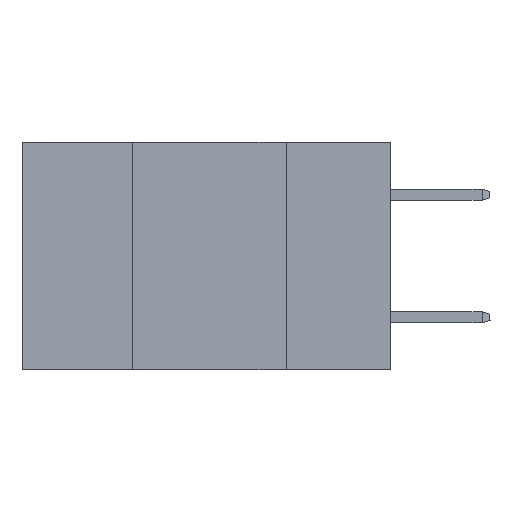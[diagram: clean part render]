
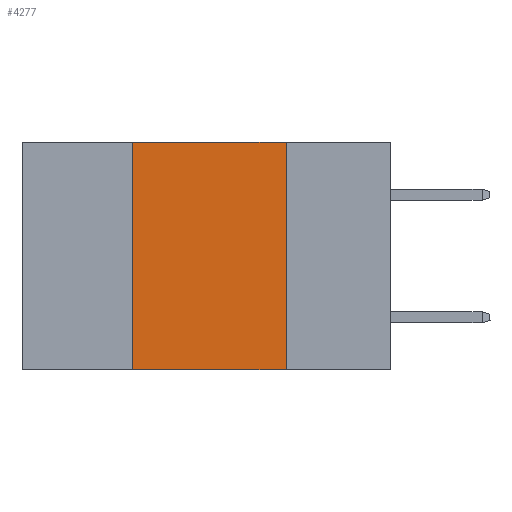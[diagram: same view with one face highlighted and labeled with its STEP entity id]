
A CAD part, left-side view. The second image highlights one B-rep face of the part: STEP entity #4277.
In plain terms, the highlighted planar face has unit normal (-1, 0, 0).
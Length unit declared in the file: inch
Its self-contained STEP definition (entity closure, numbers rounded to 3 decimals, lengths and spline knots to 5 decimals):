
#1818 = ORIENTED_EDGE ( 'NONE', *, *, #33469, .F. ) ;
#3569 = ORIENTED_EDGE ( 'NONE', *, *, #25811, .F. ) ;
#3862 = CARTESIAN_POINT ( 'NONE',  ( 0., 0.42, 0. ) ) ;
#4277 = ADVANCED_FACE ( 'NONE', ( #33760 ), #31331, .F. ) ;
#4383 = VERTEX_POINT ( 'NONE', #25792 ) ;
#5141 = DIRECTION ( 'NONE',  ( 1., 0., 0. ) ) ;
#5299 = VECTOR ( 'NONE', #25717, 39.37008 ) ;
#6858 = CARTESIAN_POINT ( 'NONE',  ( 0., 0.17, -0.37 ) ) ;
#7224 = DIRECTION ( 'NONE',  ( 0., 0., -1. ) ) ;
#7394 = CARTESIAN_POINT ( 'NONE',  ( 0., 0.6, 0. ) ) ;
#8950 = VECTOR ( 'NONE', #29360, 39.37008 ) ;
#11334 = EDGE_CURVE ( 'NONE', #19091, #15629, #13401, .T. ) ;
#11374 = ORIENTED_EDGE ( 'NONE', *, *, #11386, .T. ) ;
#11386 = EDGE_CURVE ( 'NONE', #4383, #15629, #20573, .T. ) ;
#12196 = LINE ( 'NONE', #3862, #5299 ) ;
#13239 = CARTESIAN_POINT ( 'NONE',  ( 0., 0.6, -0.37 ) ) ;
#13401 = LINE ( 'NONE', #25621, #27210 ) ;
#14486 = ORIENTED_EDGE ( 'NONE', *, *, #11334, .F. ) ;
#15629 = VERTEX_POINT ( 'NONE', #6858 ) ;
#16868 = CARTESIAN_POINT ( 'NONE',  ( 0., 0.17, 0. ) ) ;
#17795 = DIRECTION ( 'NONE',  ( 0., 0., -1. ) ) ;
#18515 = AXIS2_PLACEMENT_3D ( 'NONE', #7394, #5141, #7224 ) ;
#19091 = VERTEX_POINT ( 'NONE', #16868 ) ;
#20573 = LINE ( 'NONE', #13239, #8950 ) ;
#22776 = VECTOR ( 'NONE', #33843, 39.37008 ) ;
#23266 = LINE ( 'NONE', #28310, #22776 ) ;
#23921 = VERTEX_POINT ( 'NONE', #33021 ) ;
#25621 = CARTESIAN_POINT ( 'NONE',  ( 0., 0.17, 0. ) ) ;
#25717 = DIRECTION ( 'NONE',  ( 0., 0., 1. ) ) ;
#25792 = CARTESIAN_POINT ( 'NONE',  ( 0., 0.42, -0.37 ) ) ;
#25811 = EDGE_CURVE ( 'NONE', #23921, #19091, #23266, .T. ) ;
#27210 = VECTOR ( 'NONE', #17795, 39.37008 ) ;
#28310 = CARTESIAN_POINT ( 'NONE',  ( 0., 0.6, 0. ) ) ;
#29360 = DIRECTION ( 'NONE',  ( 0., -1., 0. ) ) ;
#31331 = PLANE ( 'NONE',  #18515 ) ;
#33021 = CARTESIAN_POINT ( 'NONE',  ( 0., 0.42, 0. ) ) ;
#33469 = EDGE_CURVE ( 'NONE', #4383, #23921, #12196, .T. ) ;
#33760 = FACE_OUTER_BOUND ( 'NONE', #33900, .T. ) ;
#33843 = DIRECTION ( 'NONE',  ( 0., -1., 0. ) ) ;
#33900 = EDGE_LOOP ( 'NONE', ( #14486, #3569, #1818, #11374 ) ) ;
